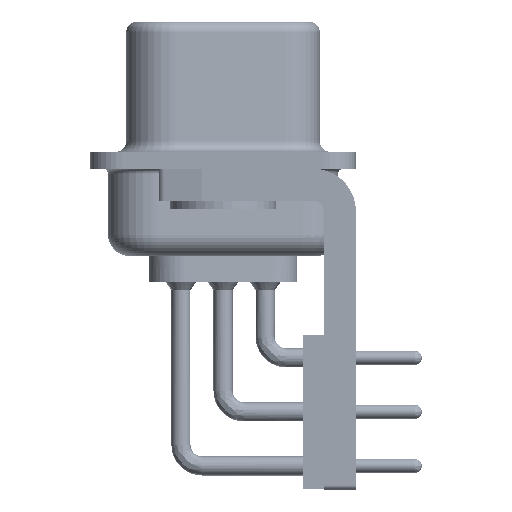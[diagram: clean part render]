
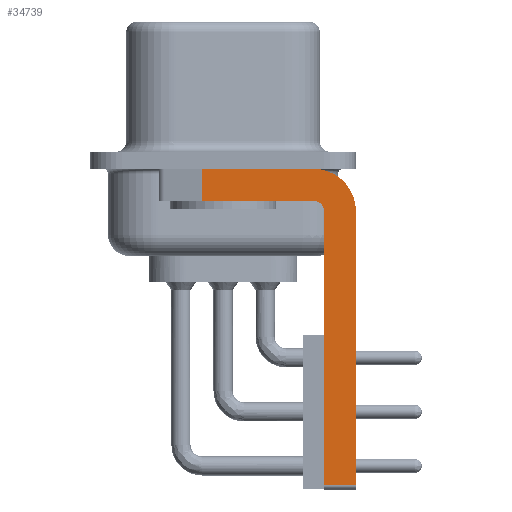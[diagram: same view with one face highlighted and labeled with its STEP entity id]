
A CAD part, left-side view. The second image highlights one B-rep face of the part: STEP entity #34739.
In plain terms, the highlighted planar face has unit normal (-1, 0, 0).
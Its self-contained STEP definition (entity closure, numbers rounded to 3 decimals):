
#719 = VECTOR ( 'NONE', #23762, 1000. ) ;
#2372 = CARTESIAN_POINT ( 'NONE',  ( -2.9, -6.25, -2.4 ) ) ;
#2521 = EDGE_CURVE ( 'NONE', #27830, #36222, #7753, .T. ) ;
#2755 = CARTESIAN_POINT ( 'NONE',  ( -2.9, -4.75, -2.4 ) ) ;
#3160 = DIRECTION ( 'NONE',  ( 1., 0., 0. ) ) ;
#3390 = CARTESIAN_POINT ( 'NONE',  ( -2.9, 0.978, -1.9 ) ) ;
#4011 = CARTESIAN_POINT ( 'NONE',  ( -2.9, -4.25, -2.4 ) ) ;
#4236 = ORIENTED_EDGE ( 'NONE', *, *, #30163, .F. ) ;
#4733 = CARTESIAN_POINT ( 'NONE',  ( -2.9, -4.25, -2.4 ) ) ;
#4811 = DIRECTION ( 'NONE',  ( 0., 0., -1. ) ) ;
#5117 = VECTOR ( 'NONE', #9837, 1000. ) ;
#5789 = EDGE_CURVE ( 'NONE', #23379, #30055, #27687, .T. ) ;
#6683 = VERTEX_POINT ( 'NONE', #36412 ) ;
#7612 = DIRECTION ( 'NONE',  ( 0., 0., 1. ) ) ;
#7753 = LINE ( 'NONE', #42990, #43357 ) ;
#7809 = VERTEX_POINT ( 'NONE', #17979 ) ;
#8334 = DIRECTION ( 'NONE',  ( 0., 0., -1. ) ) ;
#9837 = DIRECTION ( 'NONE',  ( 0., -1., 0. ) ) ;
#10199 = FACE_OUTER_BOUND ( 'NONE', #24578, .T. ) ;
#13367 = CIRCLE ( 'NONE', #33152, 2. ) ;
#14057 = VECTOR ( 'NONE', #4811, 1000. ) ;
#14611 = LINE ( 'NONE', #45301, #5117 ) ;
#15177 = LINE ( 'NONE', #33166, #14057 ) ;
#16782 = VERTEX_POINT ( 'NONE', #19934 ) ;
#17335 = DIRECTION ( 'NONE',  ( 0., 0., 1. ) ) ;
#17979 = CARTESIAN_POINT ( 'NONE',  ( -2.9, -4.25, -0.4 ) ) ;
#19214 = CARTESIAN_POINT ( 'NONE',  ( -2.9, -4.75, -15.25 ) ) ;
#19934 = CARTESIAN_POINT ( 'NONE',  ( -2.9, -6.25, -2.4 ) ) ;
#21746 = ORIENTED_EDGE ( 'NONE', *, *, #29267, .F. ) ;
#21948 = LINE ( 'NONE', #2372, #719 ) ;
#22928 = AXIS2_PLACEMENT_3D ( 'NONE', #4011, #28944, #7612 ) ;
#23191 = ORIENTED_EDGE ( 'NONE', *, *, #43347, .F. ) ;
#23379 = VERTEX_POINT ( 'NONE', #40299 ) ;
#23762 = DIRECTION ( 'NONE',  ( 0., 0., -1. ) ) ;
#24578 = EDGE_LOOP ( 'NONE', ( #21746, #45445, #32265, #4236, #34959, #38901, #34202, #23191 ) ) ;
#24616 = CARTESIAN_POINT ( 'NONE',  ( -2.9, -4.25, -1.9 ) ) ;
#25983 = VECTOR ( 'NONE', #17335, 1000. ) ;
#26169 = EDGE_CURVE ( 'NONE', #27830, #37306, #27091, .T. ) ;
#27091 = LINE ( 'NONE', #35044, #25983 ) ;
#27687 = LINE ( 'NONE', #24616, #44336 ) ;
#27830 = VERTEX_POINT ( 'NONE', #19214 ) ;
#28944 = DIRECTION ( 'NONE',  ( -1., 0., 0. ) ) ;
#29267 = EDGE_CURVE ( 'NONE', #6683, #7809, #14611, .T. ) ;
#29665 = DIRECTION ( 'NONE',  ( 1., 0., 0. ) ) ;
#29909 = DIRECTION ( 'NONE',  ( 0., -1., 0. ) ) ;
#30055 = VERTEX_POINT ( 'NONE', #3390 ) ;
#30163 = EDGE_CURVE ( 'NONE', #37306, #23379, #40156, .T. ) ;
#32265 = ORIENTED_EDGE ( 'NONE', *, *, #5789, .F. ) ;
#33152 = AXIS2_PLACEMENT_3D ( 'NONE', #4733, #29665, #8334 ) ;
#33166 = CARTESIAN_POINT ( 'NONE',  ( -2.9, 0.978, -1.9 ) ) ;
#33768 = AXIS2_PLACEMENT_3D ( 'NONE', #35408, #3160, #42548 ) ;
#34202 = ORIENTED_EDGE ( 'NONE', *, *, #34720, .F. ) ;
#34720 = EDGE_CURVE ( 'NONE', #16782, #36222, #21948, .T. ) ;
#34739 = ADVANCED_FACE ( 'NONE', ( #10199 ), #39024, .F. ) ;
#34959 = ORIENTED_EDGE ( 'NONE', *, *, #26169, .F. ) ;
#35044 = CARTESIAN_POINT ( 'NONE',  ( -2.9, -4.75, -15.5 ) ) ;
#35321 = DIRECTION ( 'NONE',  ( 0., 1., 0. ) ) ;
#35408 = CARTESIAN_POINT ( 'NONE',  ( -2.9, -4.25, -2.4 ) ) ;
#36222 = VERTEX_POINT ( 'NONE', #39331 ) ;
#36412 = CARTESIAN_POINT ( 'NONE',  ( -2.9, 0.978, -0.4 ) ) ;
#37064 = EDGE_CURVE ( 'NONE', #6683, #30055, #15177, .T. ) ;
#37306 = VERTEX_POINT ( 'NONE', #2755 ) ;
#38901 = ORIENTED_EDGE ( 'NONE', *, *, #2521, .T. ) ;
#39024 = PLANE ( 'NONE',  #33768 ) ;
#39331 = CARTESIAN_POINT ( 'NONE',  ( -2.9, -6.25, -15.25 ) ) ;
#40156 = CIRCLE ( 'NONE', #22928, 0.5 ) ;
#40299 = CARTESIAN_POINT ( 'NONE',  ( -2.9, -4.25, -1.9 ) ) ;
#42548 = DIRECTION ( 'NONE',  ( 0., 0., -1. ) ) ;
#42990 = CARTESIAN_POINT ( 'NONE',  ( -2.9, -4.25, -15.25 ) ) ;
#43347 = EDGE_CURVE ( 'NONE', #7809, #16782, #13367, .T. ) ;
#43357 = VECTOR ( 'NONE', #29909, 1000. ) ;
#44336 = VECTOR ( 'NONE', #35321, 1000. ) ;
#45301 = CARTESIAN_POINT ( 'NONE',  ( -2.9, 3., -0.4 ) ) ;
#45445 = ORIENTED_EDGE ( 'NONE', *, *, #37064, .T. ) ;
